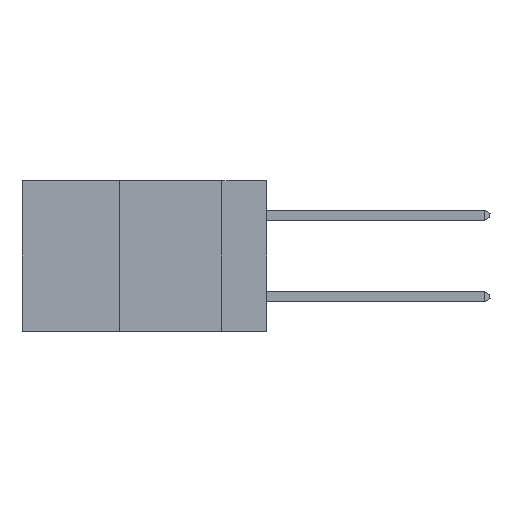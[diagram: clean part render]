
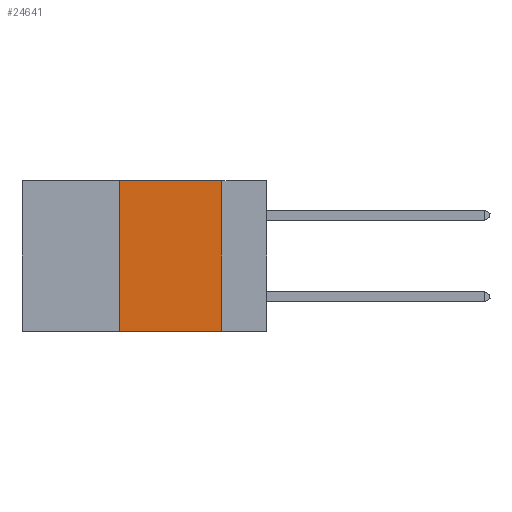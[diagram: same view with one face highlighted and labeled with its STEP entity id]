
A CAD part, left-side view. The second image highlights one B-rep face of the part: STEP entity #24641.
In plain terms, the highlighted planar face has unit normal (-1, 0, 0).
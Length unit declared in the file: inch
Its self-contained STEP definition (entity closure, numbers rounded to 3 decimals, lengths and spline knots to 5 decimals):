
#98 = DIRECTION ( 'NONE',  ( 0., 0., -1. ) ) ;
#1318 = VECTOR ( 'NONE', #21554, 39.37008 ) ;
#1360 = ORIENTED_EDGE ( 'NONE', *, *, #13424, .F. ) ;
#1673 = CARTESIAN_POINT ( 'NONE',  ( 0., 0.36, -0.37 ) ) ;
#2083 = FACE_OUTER_BOUND ( 'NONE', #37908, .T. ) ;
#2555 = CARTESIAN_POINT ( 'NONE',  ( 0., 0.6, 0. ) ) ;
#2816 = LINE ( 'NONE', #16046, #4745 ) ;
#3058 = ORIENTED_EDGE ( 'NONE', *, *, #7981, .F. ) ;
#3110 = VERTEX_POINT ( 'NONE', #1673 ) ;
#3242 = LINE ( 'NONE', #2555, #1318 ) ;
#4745 = VECTOR ( 'NONE', #31876, 39.37008 ) ;
#7981 = EDGE_CURVE ( 'NONE', #23186, #19908, #3242, .T. ) ;
#8074 = AXIS2_PLACEMENT_3D ( 'NONE', #37670, #28443, #98 ) ;
#8405 = EDGE_CURVE ( 'NONE', #19908, #8798, #25558, .T. ) ;
#8798 = VERTEX_POINT ( 'NONE', #33178 ) ;
#11055 = CARTESIAN_POINT ( 'NONE',  ( 0., 0.11, 0. ) ) ;
#11190 = DIRECTION ( 'NONE',  ( 0., 0., -1. ) ) ;
#13424 = EDGE_CURVE ( 'NONE', #3110, #23186, #22518, .T. ) ;
#16046 = CARTESIAN_POINT ( 'NONE',  ( 0., 0.6, -0.37 ) ) ;
#16931 = CARTESIAN_POINT ( 'NONE',  ( 0., 0.36, 0. ) ) ;
#19908 = VERTEX_POINT ( 'NONE', #31837 ) ;
#21554 = DIRECTION ( 'NONE',  ( 0., -1., 0. ) ) ;
#21866 = DIRECTION ( 'NONE',  ( 0., 0., 1. ) ) ;
#22518 = LINE ( 'NONE', #39498, #32202 ) ;
#23186 = VERTEX_POINT ( 'NONE', #16931 ) ;
#24641 = ADVANCED_FACE ( 'NONE', ( #2083 ), #34541, .F. ) ;
#25068 = VECTOR ( 'NONE', #11190, 39.37008 ) ;
#25558 = LINE ( 'NONE', #11055, #25068 ) ;
#25956 = ORIENTED_EDGE ( 'NONE', *, *, #8405, .F. ) ;
#28293 = EDGE_CURVE ( 'NONE', #3110, #8798, #2816, .T. ) ;
#28443 = DIRECTION ( 'NONE',  ( 1., 0., 0. ) ) ;
#31837 = CARTESIAN_POINT ( 'NONE',  ( 0., 0.11, 0. ) ) ;
#31876 = DIRECTION ( 'NONE',  ( 0., -1., 0. ) ) ;
#32202 = VECTOR ( 'NONE', #21866, 39.37008 ) ;
#33178 = CARTESIAN_POINT ( 'NONE',  ( 0., 0.11, -0.37 ) ) ;
#34541 = PLANE ( 'NONE',  #8074 ) ;
#34840 = ORIENTED_EDGE ( 'NONE', *, *, #28293, .T. ) ;
#37670 = CARTESIAN_POINT ( 'NONE',  ( 0., 0.6, 0. ) ) ;
#37908 = EDGE_LOOP ( 'NONE', ( #25956, #3058, #1360, #34840 ) ) ;
#39498 = CARTESIAN_POINT ( 'NONE',  ( 0., 0.36, 0. ) ) ;
